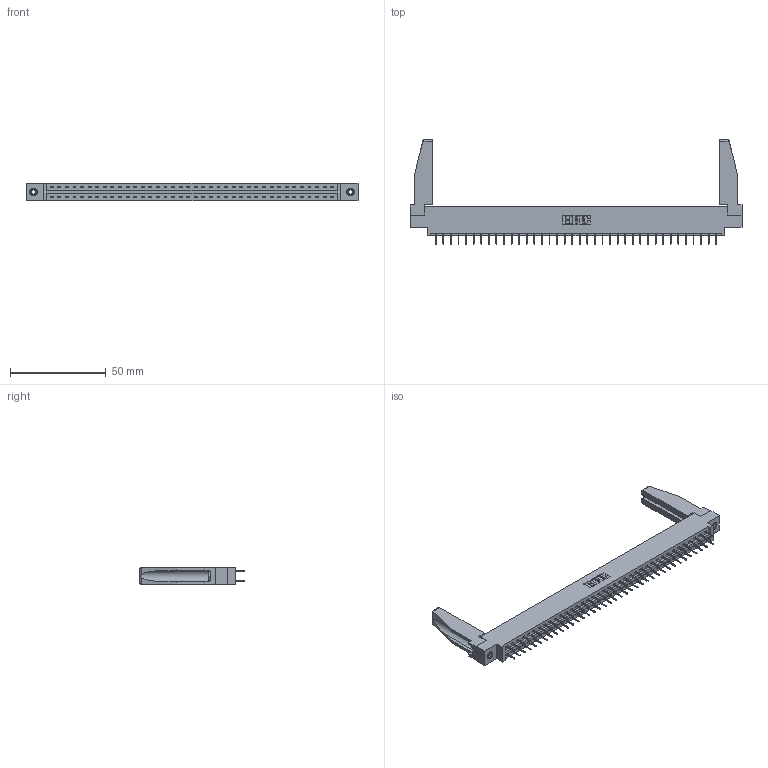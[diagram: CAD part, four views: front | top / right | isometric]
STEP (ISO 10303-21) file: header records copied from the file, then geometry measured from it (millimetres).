
FILE_DESCRIPTION (( 'STEP AP203' ), '1' );
FILE_NAME ('387-076-524-878.STEP', '2019-10-22T03:31:35', ( '' ), ( '' ), 'SwSTEP 2.0', 'SolidWorks 2016', '' );
FILE_SCHEMA (( 'CONFIG_CONTROL_DESIGN' ));
Length unit declared in the file: inch
Products named in the file (5): 345-250-001_345-250-001-102; 345-292-001_345-293-124; 307-220-078; 387-076-524-878; 337 Part_0.170 Offset - 0.156 Dia-TI
Assembly tree (81 placements, depth 2):
  387-076-524-878
    337 Part_0.170 Offset - 0.156 Dia-TI
    345-292-001_345-293-124  x76
    345-250-001_345-250-001-102  x2
    307-220-078  x2
Bounding box: 173.58 x 54.49 x 9.4 mm (x, y, z)
Volume: 22001.2 mm3; surface area: 23901.1 mm2
Topology: 81 solids, 81 shells, 4656 faces, 13193 edges, 8482 vertices
Faces by surface type: plane 3502, cylinder 1138, cone 12, torus 4
Entity records: 32626 total; most frequent: CARTESIAN_POINT 5500, ORIENTED_EDGE 5392, DIRECTION 4692, EDGE_CURVE 2696, VECTOR 2534, LINE 2534, VERTEX_POINT 1788, AXIS2_PLACEMENT_3D 1079
